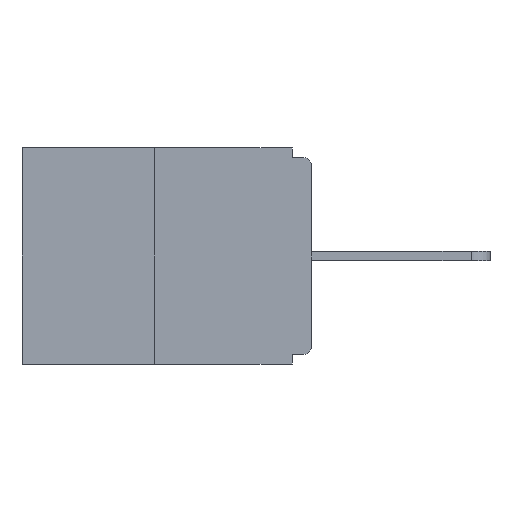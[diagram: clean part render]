
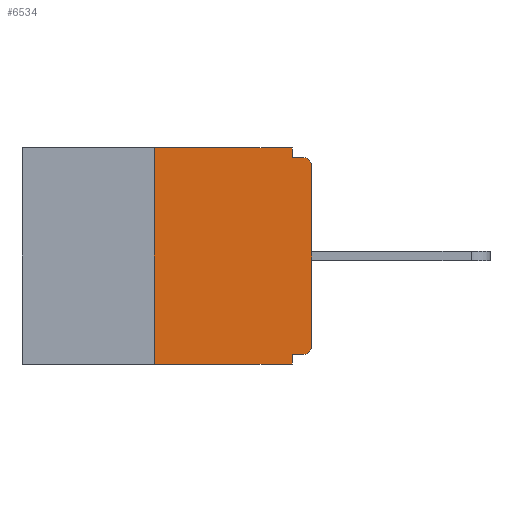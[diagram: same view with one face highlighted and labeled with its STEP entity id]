
A CAD part, left-side view. The second image highlights one B-rep face of the part: STEP entity #6534.
In plain terms, the highlighted planar face has unit normal (-1, 0, 0).
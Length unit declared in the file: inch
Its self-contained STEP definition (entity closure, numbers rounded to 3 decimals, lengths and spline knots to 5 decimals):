
#110 = EDGE_CURVE ( 'NONE', #5964, #1304, #2728, .T. ) ;
#449 = CARTESIAN_POINT ( 'NONE',  ( 0., 0., -0.015 ) ) ;
#516 = CARTESIAN_POINT ( 'NONE',  ( 0., 0.25, 0. ) ) ;
#656 = DIRECTION ( 'NONE',  ( 1., 0., 0. ) ) ;
#949 = CARTESIAN_POINT ( 'NONE',  ( 0., 0.46, -0.343 ) ) ;
#990 = CARTESIAN_POINT ( 'NONE',  ( 0., 0.031, -0.343 ) ) ;
#1207 = CARTESIAN_POINT ( 'NONE',  ( 0., 0.25, -0.343 ) ) ;
#1304 = VERTEX_POINT ( 'NONE', #2939 ) ;
#1346 = DIRECTION ( 'NONE',  ( 0., 0., -1. ) ) ;
#1433 = VERTEX_POINT ( 'NONE', #9816 ) ;
#1682 = CARTESIAN_POINT ( 'NONE',  ( 0., 0.46, 0. ) ) ;
#1735 = LINE ( 'NONE', #1682, #4008 ) ;
#1736 = ORIENTED_EDGE ( 'NONE', *, *, #8617, .F. ) ;
#1914 = EDGE_CURVE ( 'NONE', #9349, #9445, #8120, .T. ) ;
#1920 = EDGE_CURVE ( 'NONE', #7309, #6439, #4591, .T. ) ;
#2067 = DIRECTION ( 'NONE',  ( 0., 1., 0. ) ) ;
#2095 = LINE ( 'NONE', #449, #9350 ) ;
#2110 = AXIS2_PLACEMENT_3D ( 'NONE', #3083, #656, #4607 ) ;
#2195 = ORIENTED_EDGE ( 'NONE', *, *, #1920, .T. ) ;
#2524 = ORIENTED_EDGE ( 'NONE', *, *, #10362, .F. ) ;
#2537 = ORIENTED_EDGE ( 'NONE', *, *, #9965, .T. ) ;
#2610 = DIRECTION ( 'NONE',  ( 0., 0., 1. ) ) ;
#2728 = LINE ( 'NONE', #6086, #9243 ) ;
#2875 = ORIENTED_EDGE ( 'NONE', *, *, #1914, .F. ) ;
#2939 = CARTESIAN_POINT ( 'NONE',  ( 0., 0.031, -0.015 ) ) ;
#3083 = CARTESIAN_POINT ( 'NONE',  ( 0., 0.46, 0. ) ) ;
#3085 = AXIS2_PLACEMENT_3D ( 'NONE', #7430, #7323, #4966 ) ;
#3177 = VECTOR ( 'NONE', #6590, 39.37008 ) ;
#3220 = LINE ( 'NONE', #949, #9186 ) ;
#3429 = DIRECTION ( 'NONE',  ( 0., -1., 0. ) ) ;
#3496 = ORIENTED_EDGE ( 'NONE', *, *, #4441, .T. ) ;
#3800 = VERTEX_POINT ( 'NONE', #5139 ) ;
#3963 = PLANE ( 'NONE',  #2110 ) ;
#4007 = ORIENTED_EDGE ( 'NONE', *, *, #9775, .T. ) ;
#4008 = VECTOR ( 'NONE', #4911, 39.37008 ) ;
#4173 = AXIS2_PLACEMENT_3D ( 'NONE', #10337, #8760, #7077 ) ;
#4264 = CARTESIAN_POINT ( 'NONE',  ( 0., 0.031, 0. ) ) ;
#4273 = EDGE_CURVE ( 'NONE', #7309, #9053, #7646, .T. ) ;
#4441 = EDGE_CURVE ( 'NONE', #9349, #7467, #3220, .T. ) ;
#4591 = CIRCLE ( 'NONE', #3085, 0.015 ) ;
#4607 = DIRECTION ( 'NONE',  ( 0., 0., -1. ) ) ;
#4826 = ORIENTED_EDGE ( 'NONE', *, *, #110, .F. ) ;
#4898 = EDGE_CURVE ( 'NONE', #9053, #7467, #8361, .T. ) ;
#4911 = DIRECTION ( 'NONE',  ( 0., -1., 0. ) ) ;
#4966 = DIRECTION ( 'NONE',  ( 0., 0., -1. ) ) ;
#5098 = ORIENTED_EDGE ( 'NONE', *, *, #4273, .F. ) ;
#5139 = CARTESIAN_POINT ( 'NONE',  ( 0., 0., -0.03 ) ) ;
#5306 = VECTOR ( 'NONE', #2610, 39.37008 ) ;
#5353 = CARTESIAN_POINT ( 'NONE',  ( 0., 0., -0.313 ) ) ;
#5743 = CARTESIAN_POINT ( 'NONE',  ( 0., 0.25, 0. ) ) ;
#5832 = DIRECTION ( 'NONE',  ( 0., 0., -1. ) ) ;
#5928 = EDGE_LOOP ( 'NONE', ( #2524, #2875, #3496, #9665, #5098, #2195, #4007, #2537, #1736, #4826 ) ) ;
#5964 = VERTEX_POINT ( 'NONE', #4264 ) ;
#6086 = CARTESIAN_POINT ( 'NONE',  ( 0., 0.031, 0. ) ) ;
#6372 = CARTESIAN_POINT ( 'NONE',  ( 0., 0.031, -0.343 ) ) ;
#6439 = VERTEX_POINT ( 'NONE', #5353 ) ;
#6534 = ADVANCED_FACE ( 'NONE', ( #7031 ), #3963, .F. ) ;
#6590 = DIRECTION ( 'NONE',  ( 0., 0., 1. ) ) ;
#7031 = FACE_OUTER_BOUND ( 'NONE', #5928, .T. ) ;
#7077 = DIRECTION ( 'NONE',  ( 0., 0., -1. ) ) ;
#7309 = VERTEX_POINT ( 'NONE', #9482 ) ;
#7323 = DIRECTION ( 'NONE',  ( -1., 0., 0. ) ) ;
#7430 = CARTESIAN_POINT ( 'NONE',  ( 0., 0.015, -0.313 ) ) ;
#7467 = VERTEX_POINT ( 'NONE', #6372 ) ;
#7646 = LINE ( 'NONE', #9284, #9681 ) ;
#8120 = LINE ( 'NONE', #5743, #3177 ) ;
#8361 = LINE ( 'NONE', #990, #8981 ) ;
#8617 = EDGE_CURVE ( 'NONE', #1304, #1433, #2095, .T. ) ;
#8760 = DIRECTION ( 'NONE',  ( -1., 0., 0. ) ) ;
#8928 = LINE ( 'NONE', #9827, #5306 ) ;
#8981 = VECTOR ( 'NONE', #5832, 39.37008 ) ;
#9053 = VERTEX_POINT ( 'NONE', #10039 ) ;
#9186 = VECTOR ( 'NONE', #3429, 39.37008 ) ;
#9243 = VECTOR ( 'NONE', #1346, 39.37008 ) ;
#9284 = CARTESIAN_POINT ( 'NONE',  ( 0., 0., -0.328 ) ) ;
#9349 = VERTEX_POINT ( 'NONE', #1207 ) ;
#9350 = VECTOR ( 'NONE', #10154, 39.37008 ) ;
#9445 = VERTEX_POINT ( 'NONE', #516 ) ;
#9482 = CARTESIAN_POINT ( 'NONE',  ( 0., 0.015, -0.328 ) ) ;
#9665 = ORIENTED_EDGE ( 'NONE', *, *, #4898, .F. ) ;
#9681 = VECTOR ( 'NONE', #2067, 39.37008 ) ;
#9731 = CIRCLE ( 'NONE', #4173, 0.015 ) ;
#9775 = EDGE_CURVE ( 'NONE', #6439, #3800, #8928, .T. ) ;
#9816 = CARTESIAN_POINT ( 'NONE',  ( 0., 0.015, -0.015 ) ) ;
#9827 = CARTESIAN_POINT ( 'NONE',  ( 0., 0., 0. ) ) ;
#9965 = EDGE_CURVE ( 'NONE', #3800, #1433, #9731, .T. ) ;
#10039 = CARTESIAN_POINT ( 'NONE',  ( 0., 0.031, -0.328 ) ) ;
#10154 = DIRECTION ( 'NONE',  ( 0., -1., 0. ) ) ;
#10337 = CARTESIAN_POINT ( 'NONE',  ( 0., 0.015, -0.03 ) ) ;
#10362 = EDGE_CURVE ( 'NONE', #9445, #5964, #1735, .T. ) ;
